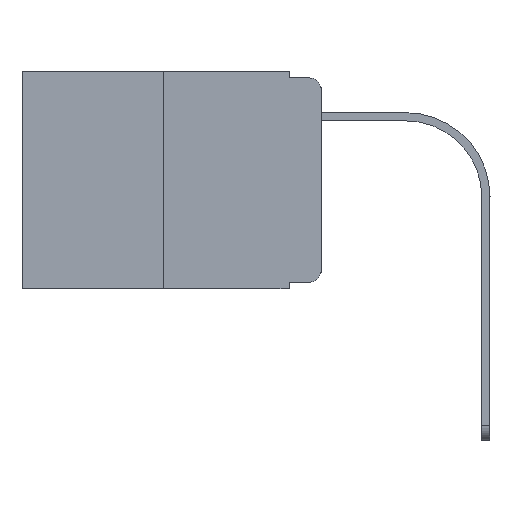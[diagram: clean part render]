
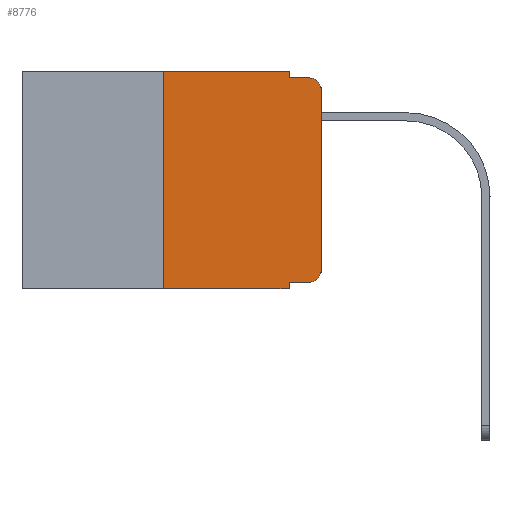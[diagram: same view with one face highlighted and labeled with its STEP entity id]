
A CAD part, left-side view. The second image highlights one B-rep face of the part: STEP entity #8776.
In plain terms, the highlighted planar face has unit normal (-1, 0, 0).
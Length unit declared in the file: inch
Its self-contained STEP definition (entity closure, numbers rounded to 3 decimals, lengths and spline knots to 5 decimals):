
#285 = EDGE_CURVE ( 'NONE', #8827, #9253, #1756, .T. ) ;
#337 = LINE ( 'NONE', #4805, #383 ) ;
#373 = ORIENTED_EDGE ( 'NONE', *, *, #8538, .F. ) ;
#383 = VECTOR ( 'NONE', #3335, 39.37008 ) ;
#464 = EDGE_CURVE ( 'NONE', #8071, #2778, #6175, .T. ) ;
#478 = EDGE_CURVE ( 'NONE', #2442, #901, #9243, .T. ) ;
#679 = CARTESIAN_POINT ( 'NONE',  ( 0., 0., -0.313 ) ) ;
#703 = VERTEX_POINT ( 'NONE', #6638 ) ;
#739 = DIRECTION ( 'NONE',  ( 0., 0., -1. ) ) ;
#901 = VERTEX_POINT ( 'NONE', #8682 ) ;
#914 = CIRCLE ( 'NONE', #3573, 0.02 ) ;
#1002 = DIRECTION ( 'NONE',  ( 0., -1., 0. ) ) ;
#1115 = PLANE ( 'NONE',  #3470 ) ;
#1123 = CARTESIAN_POINT ( 'NONE',  ( 0., 0.051, -0.333 ) ) ;
#1244 = CARTESIAN_POINT ( 'NONE',  ( 0., 0.051, 0. ) ) ;
#1401 = CARTESIAN_POINT ( 'NONE',  ( 0., 0.02, -0.03 ) ) ;
#1407 = ORIENTED_EDGE ( 'NONE', *, *, #9078, .T. ) ;
#1627 = CARTESIAN_POINT ( 'NONE',  ( 0., 0.051, 0. ) ) ;
#1685 = CARTESIAN_POINT ( 'NONE',  ( 0., 0.051, -0.333 ) ) ;
#1756 = LINE ( 'NONE', #3773, #7936 ) ;
#1842 = VECTOR ( 'NONE', #1002, 39.37008 ) ;
#2260 = CARTESIAN_POINT ( 'NONE',  ( 0., 0.25, 0. ) ) ;
#2272 = LINE ( 'NONE', #1627, #8280 ) ;
#2357 = CARTESIAN_POINT ( 'NONE',  ( 0., 0.051, -0.343 ) ) ;
#2375 = AXIS2_PLACEMENT_3D ( 'NONE', #8894, #4431, #7424 ) ;
#2427 = VECTOR ( 'NONE', #4302, 39.37008 ) ;
#2433 = CARTESIAN_POINT ( 'NONE',  ( 0., 0., 0. ) ) ;
#2442 = VERTEX_POINT ( 'NONE', #1123 ) ;
#2583 = ORIENTED_EDGE ( 'NONE', *, *, #4331, .F. ) ;
#2728 = LINE ( 'NONE', #1244, #2427 ) ;
#2778 = VERTEX_POINT ( 'NONE', #7186 ) ;
#3241 = DIRECTION ( 'NONE',  ( 0., -1., 0. ) ) ;
#3260 = EDGE_CURVE ( 'NONE', #2442, #7699, #2728, .T. ) ;
#3335 = DIRECTION ( 'NONE',  ( 0., -1., 0. ) ) ;
#3349 = VECTOR ( 'NONE', #7887, 39.37008 ) ;
#3470 = AXIS2_PLACEMENT_3D ( 'NONE', #6424, #6469, #8031 ) ;
#3471 = FACE_OUTER_BOUND ( 'NONE', #7857, .T. ) ;
#3573 = AXIS2_PLACEMENT_3D ( 'NONE', #1401, #7406, #739 ) ;
#3773 = CARTESIAN_POINT ( 'NONE',  ( 0., 0.25, 0. ) ) ;
#3848 = VECTOR ( 'NONE', #3241, 39.37008 ) ;
#3905 = CARTESIAN_POINT ( 'NONE',  ( 0., 0.02, -0.01 ) ) ;
#4221 = LINE ( 'NONE', #9373, #3349 ) ;
#4302 = DIRECTION ( 'NONE',  ( 0., 0., -1. ) ) ;
#4331 = EDGE_CURVE ( 'NONE', #703, #5867, #337, .T. ) ;
#4431 = DIRECTION ( 'NONE',  ( -1., 0., 0. ) ) ;
#4438 = EDGE_CURVE ( 'NONE', #8827, #7699, #9173, .T. ) ;
#4666 = DIRECTION ( 'NONE',  ( 0., 0., 1. ) ) ;
#4805 = CARTESIAN_POINT ( 'NONE',  ( 0., 0.051, -0.01 ) ) ;
#4889 = CARTESIAN_POINT ( 'NONE',  ( 0., 0.25, -0.343 ) ) ;
#5385 = CARTESIAN_POINT ( 'NONE',  ( 0., 0.051, 0. ) ) ;
#5823 = ORIENTED_EDGE ( 'NONE', *, *, #478, .T. ) ;
#5867 = VERTEX_POINT ( 'NONE', #3905 ) ;
#6175 = LINE ( 'NONE', #2433, #7807 ) ;
#6311 = DIRECTION ( 'NONE',  ( 0., 0., 1. ) ) ;
#6424 = CARTESIAN_POINT ( 'NONE',  ( 0., 0.473, 0. ) ) ;
#6442 = EDGE_CURVE ( 'NONE', #2778, #5867, #914, .T. ) ;
#6469 = DIRECTION ( 'NONE',  ( 1., 0., 0. ) ) ;
#6565 = VERTEX_POINT ( 'NONE', #5385 ) ;
#6612 = CIRCLE ( 'NONE', #2375, 0.02 ) ;
#6638 = CARTESIAN_POINT ( 'NONE',  ( 0., 0.051, -0.01 ) ) ;
#6681 = EDGE_CURVE ( 'NONE', #6565, #703, #2272, .T. ) ;
#7186 = CARTESIAN_POINT ( 'NONE',  ( 0., 0., -0.03 ) ) ;
#7406 = DIRECTION ( 'NONE',  ( -1., 0., 0. ) ) ;
#7424 = DIRECTION ( 'NONE',  ( 0., 0., -1. ) ) ;
#7643 = ORIENTED_EDGE ( 'NONE', *, *, #464, .T. ) ;
#7699 = VERTEX_POINT ( 'NONE', #2357 ) ;
#7807 = VECTOR ( 'NONE', #6311, 39.37008 ) ;
#7857 = EDGE_LOOP ( 'NONE', ( #7643, #8082, #2583, #8703, #373, #9674, #8525, #8326, #5823, #1407 ) ) ;
#7887 = DIRECTION ( 'NONE',  ( 0., -1., 0. ) ) ;
#7936 = VECTOR ( 'NONE', #4666, 39.37008 ) ;
#8031 = DIRECTION ( 'NONE',  ( 0., 0., -1. ) ) ;
#8071 = VERTEX_POINT ( 'NONE', #679 ) ;
#8082 = ORIENTED_EDGE ( 'NONE', *, *, #6442, .T. ) ;
#8280 = VECTOR ( 'NONE', #9091, 39.37008 ) ;
#8326 = ORIENTED_EDGE ( 'NONE', *, *, #3260, .F. ) ;
#8525 = ORIENTED_EDGE ( 'NONE', *, *, #4438, .T. ) ;
#8538 = EDGE_CURVE ( 'NONE', #9253, #6565, #4221, .T. ) ;
#8682 = CARTESIAN_POINT ( 'NONE',  ( 0., 0.02, -0.333 ) ) ;
#8703 = ORIENTED_EDGE ( 'NONE', *, *, #6681, .F. ) ;
#8776 = ADVANCED_FACE ( 'NONE', ( #3471 ), #1115, .F. ) ;
#8827 = VERTEX_POINT ( 'NONE', #4889 ) ;
#8894 = CARTESIAN_POINT ( 'NONE',  ( 0., 0.02, -0.313 ) ) ;
#9078 = EDGE_CURVE ( 'NONE', #901, #8071, #6612, .T. ) ;
#9091 = DIRECTION ( 'NONE',  ( 0., 0., -1. ) ) ;
#9173 = LINE ( 'NONE', #9370, #3848 ) ;
#9243 = LINE ( 'NONE', #1685, #1842 ) ;
#9253 = VERTEX_POINT ( 'NONE', #2260 ) ;
#9370 = CARTESIAN_POINT ( 'NONE',  ( 0., 0.473, -0.343 ) ) ;
#9373 = CARTESIAN_POINT ( 'NONE',  ( 0., 0.473, 0. ) ) ;
#9674 = ORIENTED_EDGE ( 'NONE', *, *, #285, .F. ) ;
